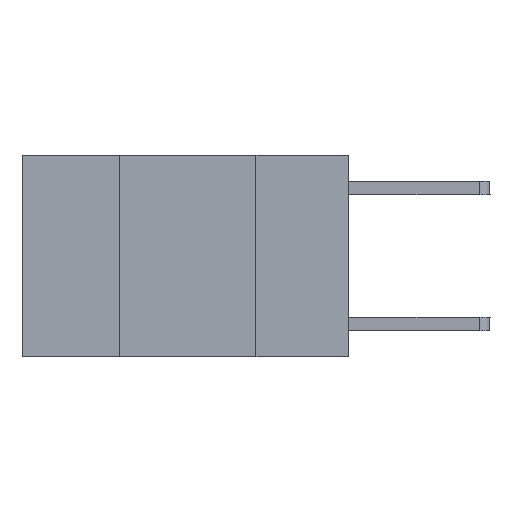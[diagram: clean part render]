
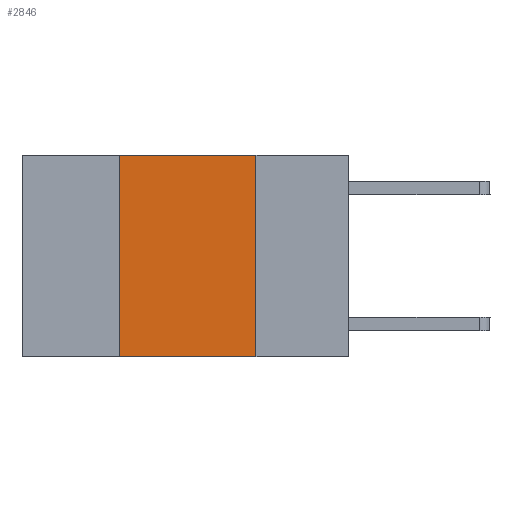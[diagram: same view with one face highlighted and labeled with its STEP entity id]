
A CAD part, left-side view. The second image highlights one B-rep face of the part: STEP entity #2846.
In plain terms, the highlighted planar face has unit normal (-1, 0, 0).
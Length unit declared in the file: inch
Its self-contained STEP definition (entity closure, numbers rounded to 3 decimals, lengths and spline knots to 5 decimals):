
#275 = VERTEX_POINT ( 'NONE', #9330 ) ;
#574 = ORIENTED_EDGE ( 'NONE', *, *, #3933, .F. ) ;
#667 = VECTOR ( 'NONE', #3375, 39.37008 ) ;
#718 = DIRECTION ( 'NONE',  ( 0., 0., -1. ) ) ;
#907 = CARTESIAN_POINT ( 'NONE',  ( 0., 0.6, 0. ) ) ;
#933 = CARTESIAN_POINT ( 'NONE',  ( 0., 0.17, 0. ) ) ;
#1665 = CARTESIAN_POINT ( 'NONE',  ( 0., 0.42, 0. ) ) ;
#1733 = DIRECTION ( 'NONE',  ( 1., 0., 0. ) ) ;
#1803 = VERTEX_POINT ( 'NONE', #4126 ) ;
#2600 = EDGE_LOOP ( 'NONE', ( #574, #2655, #4429, #3584 ) ) ;
#2655 = ORIENTED_EDGE ( 'NONE', *, *, #5047, .F. ) ;
#2846 = ADVANCED_FACE ( 'NONE', ( #3512 ), #8801, .F. ) ;
#3375 = DIRECTION ( 'NONE',  ( 0., -1., 0. ) ) ;
#3483 = LINE ( 'NONE', #7739, #667 ) ;
#3512 = FACE_OUTER_BOUND ( 'NONE', #2600, .T. ) ;
#3584 = ORIENTED_EDGE ( 'NONE', *, *, #7489, .T. ) ;
#3826 = LINE ( 'NONE', #10098, #4170 ) ;
#3933 = EDGE_CURVE ( 'NONE', #7059, #275, #8709, .T. ) ;
#4126 = CARTESIAN_POINT ( 'NONE',  ( 0., 0.42, 0. ) ) ;
#4170 = VECTOR ( 'NONE', #4595, 39.37008 ) ;
#4177 = VECTOR ( 'NONE', #9795, 39.37008 ) ;
#4216 = CARTESIAN_POINT ( 'NONE',  ( 0., 0.17, 0. ) ) ;
#4429 = ORIENTED_EDGE ( 'NONE', *, *, #7805, .F. ) ;
#4455 = CARTESIAN_POINT ( 'NONE',  ( 0., 0.42, -0.37 ) ) ;
#4595 = DIRECTION ( 'NONE',  ( 0., -1., 0. ) ) ;
#5047 = EDGE_CURVE ( 'NONE', #1803, #7059, #3483, .T. ) ;
#6189 = LINE ( 'NONE', #1665, #4177 ) ;
#6851 = DIRECTION ( 'NONE',  ( 0., 0., -1. ) ) ;
#7059 = VERTEX_POINT ( 'NONE', #933 ) ;
#7489 = EDGE_CURVE ( 'NONE', #9709, #275, #3826, .T. ) ;
#7739 = CARTESIAN_POINT ( 'NONE',  ( 0., 0.6, 0. ) ) ;
#7805 = EDGE_CURVE ( 'NONE', #9709, #1803, #6189, .T. ) ;
#8709 = LINE ( 'NONE', #4216, #9981 ) ;
#8801 = PLANE ( 'NONE',  #10938 ) ;
#9330 = CARTESIAN_POINT ( 'NONE',  ( 0., 0.17, -0.37 ) ) ;
#9709 = VERTEX_POINT ( 'NONE', #4455 ) ;
#9795 = DIRECTION ( 'NONE',  ( 0., 0., 1. ) ) ;
#9981 = VECTOR ( 'NONE', #718, 39.37008 ) ;
#10098 = CARTESIAN_POINT ( 'NONE',  ( 0., 0.6, -0.37 ) ) ;
#10938 = AXIS2_PLACEMENT_3D ( 'NONE', #907, #1733, #6851 ) ;
